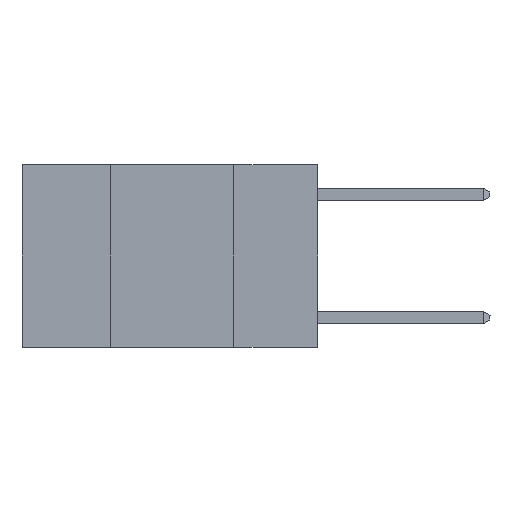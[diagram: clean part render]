
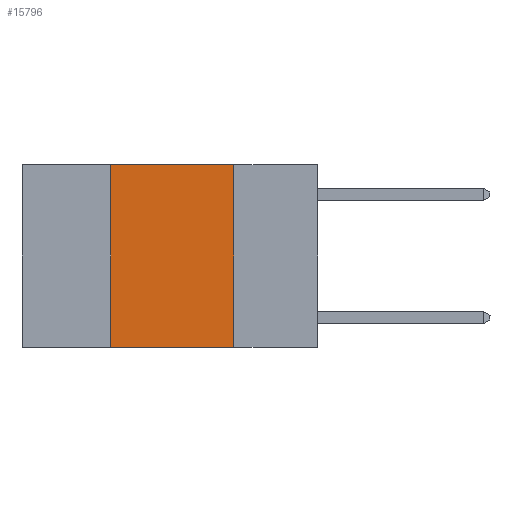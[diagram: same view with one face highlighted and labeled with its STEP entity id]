
A CAD part, left-side view. The second image highlights one B-rep face of the part: STEP entity #15796.
In plain terms, the highlighted planar face has unit normal (-1, 0, 0).
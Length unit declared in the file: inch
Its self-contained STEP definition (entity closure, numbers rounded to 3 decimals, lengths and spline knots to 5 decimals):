
#95 = DIRECTION ( 'NONE',  ( 0., -1., 0. ) ) ;
#108 = CARTESIAN_POINT ( 'NONE',  ( 0., 0.17, -0.37 ) ) ;
#1090 = LINE ( 'NONE', #13965, #13331 ) ;
#2195 = VERTEX_POINT ( 'NONE', #108 ) ;
#2894 = VECTOR ( 'NONE', #25342, 39.37008 ) ;
#4334 = LINE ( 'NONE', #14755, #9277 ) ;
#6830 = CARTESIAN_POINT ( 'NONE',  ( 0., 0.42, -0.37 ) ) ;
#8431 = VERTEX_POINT ( 'NONE', #21856 ) ;
#9186 = CARTESIAN_POINT ( 'NONE',  ( 0., 0.6, 0. ) ) ;
#9277 = VECTOR ( 'NONE', #95, 39.37008 ) ;
#10630 = VERTEX_POINT ( 'NONE', #6830 ) ;
#10923 = LINE ( 'NONE', #13291, #2894 ) ;
#11364 = LINE ( 'NONE', #14647, #17071 ) ;
#11473 = VERTEX_POINT ( 'NONE', #14711 ) ;
#12207 = ORIENTED_EDGE ( 'NONE', *, *, #27758, .F. ) ;
#13291 = CARTESIAN_POINT ( 'NONE',  ( 0., 0.42, 0. ) ) ;
#13331 = VECTOR ( 'NONE', #18819, 39.37008 ) ;
#13965 = CARTESIAN_POINT ( 'NONE',  ( 0., 0.6, 0. ) ) ;
#14270 = DIRECTION ( 'NONE',  ( 0., 0., -1. ) ) ;
#14571 = EDGE_LOOP ( 'NONE', ( #15634, #29928, #12207, #18621 ) ) ;
#14647 = CARTESIAN_POINT ( 'NONE',  ( 0., 0.17, 0. ) ) ;
#14711 = CARTESIAN_POINT ( 'NONE',  ( 0., 0.42, 0. ) ) ;
#14755 = CARTESIAN_POINT ( 'NONE',  ( 0., 0.6, -0.37 ) ) ;
#15634 = ORIENTED_EDGE ( 'NONE', *, *, #18526, .F. ) ;
#15796 = ADVANCED_FACE ( 'NONE', ( #25002 ), #26304, .F. ) ;
#17071 = VECTOR ( 'NONE', #29056, 39.37008 ) ;
#17089 = EDGE_CURVE ( 'NONE', #11473, #8431, #1090, .T. ) ;
#17520 = AXIS2_PLACEMENT_3D ( 'NONE', #9186, #28697, #14270 ) ;
#18526 = EDGE_CURVE ( 'NONE', #8431, #2195, #11364, .T. ) ;
#18621 = ORIENTED_EDGE ( 'NONE', *, *, #20693, .T. ) ;
#18819 = DIRECTION ( 'NONE',  ( 0., -1., 0. ) ) ;
#20693 = EDGE_CURVE ( 'NONE', #10630, #2195, #4334, .T. ) ;
#21856 = CARTESIAN_POINT ( 'NONE',  ( 0., 0.17, 0. ) ) ;
#25002 = FACE_OUTER_BOUND ( 'NONE', #14571, .T. ) ;
#25342 = DIRECTION ( 'NONE',  ( 0., 0., 1. ) ) ;
#26304 = PLANE ( 'NONE',  #17520 ) ;
#27758 = EDGE_CURVE ( 'NONE', #10630, #11473, #10923, .T. ) ;
#28697 = DIRECTION ( 'NONE',  ( 1., 0., 0. ) ) ;
#29056 = DIRECTION ( 'NONE',  ( 0., 0., -1. ) ) ;
#29928 = ORIENTED_EDGE ( 'NONE', *, *, #17089, .F. ) ;
